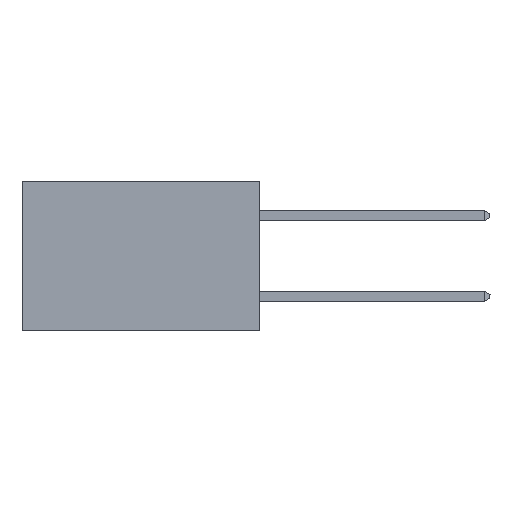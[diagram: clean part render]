
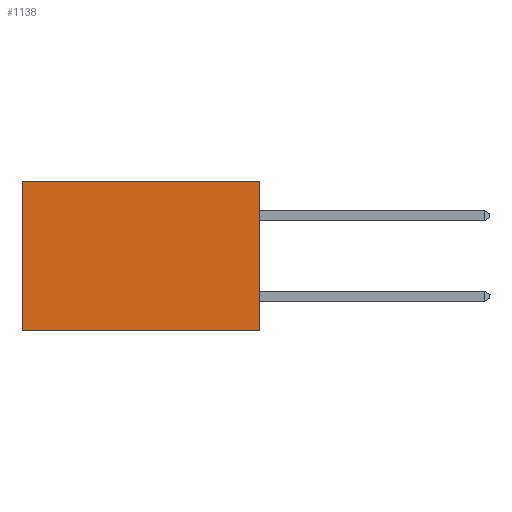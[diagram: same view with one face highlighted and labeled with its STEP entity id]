
A CAD part, left-side view. The second image highlights one B-rep face of the part: STEP entity #1138.
In plain terms, the highlighted planar face has unit normal (-1, 0, 0).
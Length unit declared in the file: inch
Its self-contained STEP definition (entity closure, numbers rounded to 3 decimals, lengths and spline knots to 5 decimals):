
#240 = LINE ( 'NONE', #7097, #5639 ) ;
#704 = EDGE_CURVE ( 'NONE', #5840, #2744, #2046, .T. ) ;
#949 = EDGE_CURVE ( 'NONE', #8006, #2744, #240, .T. ) ;
#1036 = ORIENTED_EDGE ( 'NONE', *, *, #949, .T. ) ;
#1138 = ADVANCED_FACE ( 'NONE', ( #8576 ), #3348, .F. ) ;
#1278 = ORIENTED_EDGE ( 'NONE', *, *, #5097, .T. ) ;
#1349 = DIRECTION ( 'NONE',  ( 0., 0., -1. ) ) ;
#1393 = CARTESIAN_POINT ( 'NONE',  ( 0.277, 0., -0.37 ) ) ;
#1445 = DIRECTION ( 'NONE',  ( 0., 0., -1. ) ) ;
#2046 = LINE ( 'NONE', #5348, #2375 ) ;
#2375 = VECTOR ( 'NONE', #6356, 39.37008 ) ;
#2703 = VECTOR ( 'NONE', #7386, 39.37008 ) ;
#2744 = VERTEX_POINT ( 'NONE', #6975 ) ;
#2889 = ORIENTED_EDGE ( 'NONE', *, *, #704, .F. ) ;
#3348 = PLANE ( 'NONE',  #9416 ) ;
#3610 = CARTESIAN_POINT ( 'NONE',  ( 0.277, 0., 0. ) ) ;
#3663 = CARTESIAN_POINT ( 'NONE',  ( 0.277, 0., -0.37 ) ) ;
#3876 = CARTESIAN_POINT ( 'NONE',  ( 0.277, 0.59, 0. ) ) ;
#4070 = DIRECTION ( 'NONE',  ( 0., 0., -1. ) ) ;
#4164 = DIRECTION ( 'NONE',  ( 1., 0., 0. ) ) ;
#4350 = VERTEX_POINT ( 'NONE', #4599 ) ;
#4599 = CARTESIAN_POINT ( 'NONE',  ( 0.277, 0., 0. ) ) ;
#5097 = EDGE_CURVE ( 'NONE', #4350, #8006, #8616, .T. ) ;
#5205 = CARTESIAN_POINT ( 'NONE',  ( 0.277, 0., -0.37 ) ) ;
#5348 = CARTESIAN_POINT ( 'NONE',  ( 0.277, 0., -0.37 ) ) ;
#5639 = VECTOR ( 'NONE', #1445, 39.37008 ) ;
#5777 = VECTOR ( 'NONE', #1349, 39.37008 ) ;
#5840 = VERTEX_POINT ( 'NONE', #3663 ) ;
#6356 = DIRECTION ( 'NONE',  ( 0., 1., 0. ) ) ;
#6794 = EDGE_CURVE ( 'NONE', #4350, #5840, #7788, .T. ) ;
#6848 = ORIENTED_EDGE ( 'NONE', *, *, #6794, .F. ) ;
#6975 = CARTESIAN_POINT ( 'NONE',  ( 0.277, 0.59, -0.37 ) ) ;
#7097 = CARTESIAN_POINT ( 'NONE',  ( 0.277, 0.59, -0.37 ) ) ;
#7386 = DIRECTION ( 'NONE',  ( 0., 1., 0. ) ) ;
#7460 = EDGE_LOOP ( 'NONE', ( #1036, #2889, #6848, #1278 ) ) ;
#7788 = LINE ( 'NONE', #1393, #5777 ) ;
#8006 = VERTEX_POINT ( 'NONE', #3876 ) ;
#8576 = FACE_OUTER_BOUND ( 'NONE', #7460, .T. ) ;
#8616 = LINE ( 'NONE', #3610, #2703 ) ;
#9416 = AXIS2_PLACEMENT_3D ( 'NONE', #5205, #4164, #4070 ) ;
